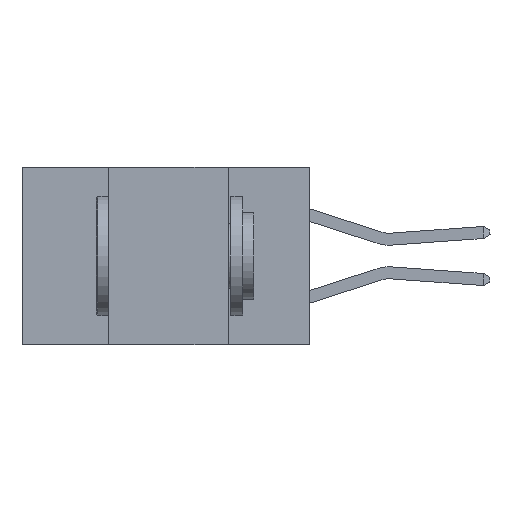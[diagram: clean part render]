
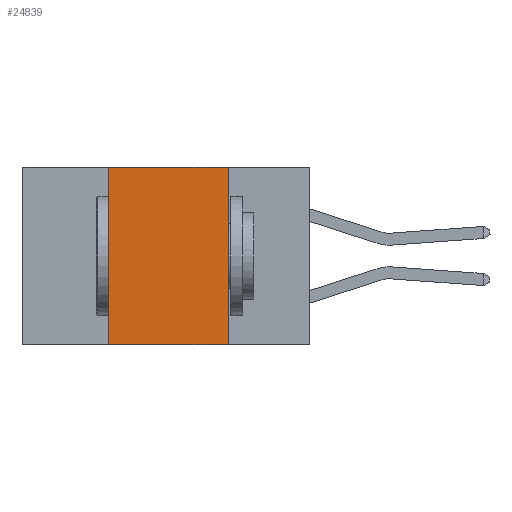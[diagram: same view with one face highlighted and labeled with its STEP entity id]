
A CAD part, left-side view. The second image highlights one B-rep face of the part: STEP entity #24839.
In plain terms, the highlighted planar face has unit normal (-1, 0, 0).
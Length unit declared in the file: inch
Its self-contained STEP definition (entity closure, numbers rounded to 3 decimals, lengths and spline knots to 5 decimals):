
#964 = EDGE_CURVE ( 'NONE', #9808, #30161, #30197, .T. ) ;
#1064 = VERTEX_POINT ( 'NONE', #23022 ) ;
#3979 = PLANE ( 'NONE',  #8805 ) ;
#4392 = VECTOR ( 'NONE', #19624, 39.37008 ) ;
#4712 = VECTOR ( 'NONE', #16809, 39.37008 ) ;
#5157 = LINE ( 'NONE', #8230, #4392 ) ;
#5661 = ORIENTED_EDGE ( 'NONE', *, *, #17370, .F. ) ;
#8230 = CARTESIAN_POINT ( 'NONE',  ( 0., 0.17, 0. ) ) ;
#8805 = AXIS2_PLACEMENT_3D ( 'NONE', #11041, #27293, #13301 ) ;
#9808 = VERTEX_POINT ( 'NONE', #13134 ) ;
#10345 = CARTESIAN_POINT ( 'NONE',  ( 0., 0.42, 0. ) ) ;
#11026 = EDGE_CURVE ( 'NONE', #1064, #30161, #5157, .T. ) ;
#11041 = CARTESIAN_POINT ( 'NONE',  ( 0., 0.6, 0. ) ) ;
#11809 = VECTOR ( 'NONE', #12991, 39.37008 ) ;
#12227 = CARTESIAN_POINT ( 'NONE',  ( 0., 0.6, 0. ) ) ;
#12361 = VECTOR ( 'NONE', #14945, 39.37008 ) ;
#12528 = ORIENTED_EDGE ( 'NONE', *, *, #964, .T. ) ;
#12991 = DIRECTION ( 'NONE',  ( 0., 0., 1. ) ) ;
#13134 = CARTESIAN_POINT ( 'NONE',  ( 0., 0.42, -0.37 ) ) ;
#13301 = DIRECTION ( 'NONE',  ( 0., 0., -1. ) ) ;
#14774 = EDGE_CURVE ( 'NONE', #9808, #22199, #24825, .T. ) ;
#14815 = CARTESIAN_POINT ( 'NONE',  ( 0., 0.6, -0.37 ) ) ;
#14945 = DIRECTION ( 'NONE',  ( 0., -1., 0. ) ) ;
#16809 = DIRECTION ( 'NONE',  ( 0., -1., 0. ) ) ;
#16990 = LINE ( 'NONE', #12227, #4712 ) ;
#17073 = CARTESIAN_POINT ( 'NONE',  ( 0., 0.17, -0.37 ) ) ;
#17370 = EDGE_CURVE ( 'NONE', #22199, #1064, #16990, .T. ) ;
#17757 = EDGE_LOOP ( 'NONE', ( #22666, #5661, #17903, #12528 ) ) ;
#17903 = ORIENTED_EDGE ( 'NONE', *, *, #14774, .F. ) ;
#19096 = FACE_OUTER_BOUND ( 'NONE', #17757, .T. ) ;
#19624 = DIRECTION ( 'NONE',  ( 0., 0., -1. ) ) ;
#22199 = VERTEX_POINT ( 'NONE', #10345 ) ;
#22666 = ORIENTED_EDGE ( 'NONE', *, *, #11026, .F. ) ;
#23022 = CARTESIAN_POINT ( 'NONE',  ( 0., 0.17, 0. ) ) ;
#24564 = CARTESIAN_POINT ( 'NONE',  ( 0., 0.42, 0. ) ) ;
#24825 = LINE ( 'NONE', #24564, #11809 ) ;
#24839 = ADVANCED_FACE ( 'NONE', ( #19096 ), #3979, .F. ) ;
#27293 = DIRECTION ( 'NONE',  ( 1., 0., 0. ) ) ;
#30161 = VERTEX_POINT ( 'NONE', #17073 ) ;
#30197 = LINE ( 'NONE', #14815, #12361 ) ;
